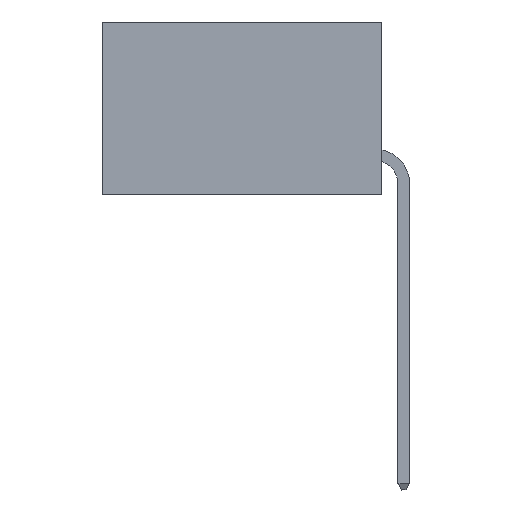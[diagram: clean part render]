
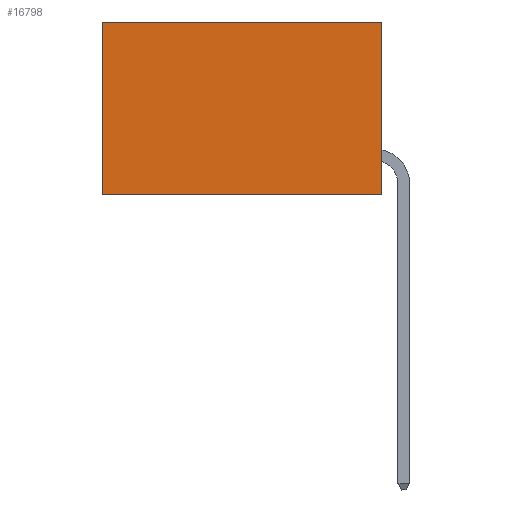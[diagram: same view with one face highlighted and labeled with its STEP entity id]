
A CAD part, left-side view. The second image highlights one B-rep face of the part: STEP entity #16798.
In plain terms, the highlighted planar face has unit normal (-1, 0, 0).
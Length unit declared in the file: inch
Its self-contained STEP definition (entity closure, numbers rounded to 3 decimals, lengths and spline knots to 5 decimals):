
#507 = EDGE_CURVE ( 'NONE', #31940, #26035, #16235, .T. ) ;
#909 = CARTESIAN_POINT ( 'NONE',  ( 0.2875, 0., -0.37 ) ) ;
#1222 = DIRECTION ( 'NONE',  ( 0., 0., -1. ) ) ;
#4314 = CARTESIAN_POINT ( 'NONE',  ( 0.2875, 0.6, 0. ) ) ;
#4966 = VECTOR ( 'NONE', #6521, 39.37008 ) ;
#5840 = CARTESIAN_POINT ( 'NONE',  ( 0.2875, 0.6, 0. ) ) ;
#5852 = VECTOR ( 'NONE', #13963, 39.37008 ) ;
#6521 = DIRECTION ( 'NONE',  ( 0., 1., 0. ) ) ;
#8524 = LINE ( 'NONE', #27493, #5852 ) ;
#10147 = LINE ( 'NONE', #27461, #24046 ) ;
#11689 = CARTESIAN_POINT ( 'NONE',  ( 0.2875, 0., 0. ) ) ;
#11795 = LINE ( 'NONE', #5840, #17665 ) ;
#13103 = VERTEX_POINT ( 'NONE', #29390 ) ;
#13586 = EDGE_LOOP ( 'NONE', ( #17176, #26381, #23925, #15532 ) ) ;
#13796 = DIRECTION ( 'NONE',  ( 0., 1., 0. ) ) ;
#13963 = DIRECTION ( 'NONE',  ( 0., 0., -1. ) ) ;
#15532 = ORIENTED_EDGE ( 'NONE', *, *, #507, .T. ) ;
#16235 = LINE ( 'NONE', #17090, #4966 ) ;
#16798 = ADVANCED_FACE ( 'NONE', ( #28856 ), #31756, .F. ) ;
#17090 = CARTESIAN_POINT ( 'NONE',  ( 0.2875, 0., 0. ) ) ;
#17143 = CARTESIAN_POINT ( 'NONE',  ( 0.2875, 0., 0. ) ) ;
#17176 = ORIENTED_EDGE ( 'NONE', *, *, #35932, .T. ) ;
#17665 = VECTOR ( 'NONE', #29188, 39.37008 ) ;
#22756 = EDGE_CURVE ( 'NONE', #31940, #31522, #8524, .T. ) ;
#23925 = ORIENTED_EDGE ( 'NONE', *, *, #22756, .F. ) ;
#24046 = VECTOR ( 'NONE', #13796, 39.37008 ) ;
#24591 = AXIS2_PLACEMENT_3D ( 'NONE', #11689, #25489, #1222 ) ;
#25231 = EDGE_CURVE ( 'NONE', #31522, #13103, #10147, .T. ) ;
#25489 = DIRECTION ( 'NONE',  ( 1., 0., 0. ) ) ;
#26035 = VERTEX_POINT ( 'NONE', #4314 ) ;
#26381 = ORIENTED_EDGE ( 'NONE', *, *, #25231, .F. ) ;
#27461 = CARTESIAN_POINT ( 'NONE',  ( 0.2875, 0., -0.37 ) ) ;
#27493 = CARTESIAN_POINT ( 'NONE',  ( 0.2875, 0., 0. ) ) ;
#28856 = FACE_OUTER_BOUND ( 'NONE', #13586, .T. ) ;
#29188 = DIRECTION ( 'NONE',  ( 0., 0., -1. ) ) ;
#29390 = CARTESIAN_POINT ( 'NONE',  ( 0.2875, 0.6, -0.37 ) ) ;
#31522 = VERTEX_POINT ( 'NONE', #909 ) ;
#31756 = PLANE ( 'NONE',  #24591 ) ;
#31940 = VERTEX_POINT ( 'NONE', #17143 ) ;
#35932 = EDGE_CURVE ( 'NONE', #26035, #13103, #11795, .T. ) ;
